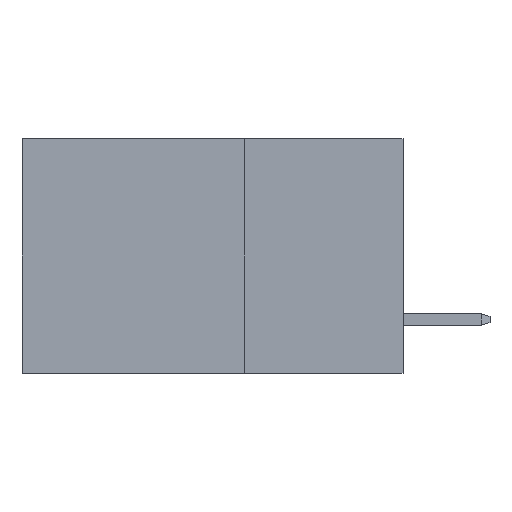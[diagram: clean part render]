
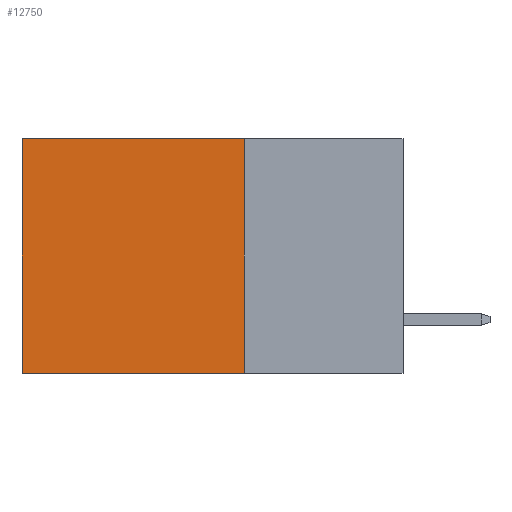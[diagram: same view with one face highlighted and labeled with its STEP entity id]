
A CAD part, left-side view. The second image highlights one B-rep face of the part: STEP entity #12750.
In plain terms, the highlighted planar face has unit normal (-1, 0, 0).
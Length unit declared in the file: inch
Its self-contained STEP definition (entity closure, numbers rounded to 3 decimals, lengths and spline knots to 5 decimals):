
#389 = VERTEX_POINT ( 'NONE', #21893 ) ;
#2027 = CARTESIAN_POINT ( 'NONE',  ( 0.2875, 0.25, 0. ) ) ;
#3282 = VECTOR ( 'NONE', #28069, 39.37008 ) ;
#3759 = EDGE_LOOP ( 'NONE', ( #11251, #27852, #19115, #13332 ) ) ;
#3894 = DIRECTION ( 'NONE',  ( 0., 0., -1. ) ) ;
#3931 = CARTESIAN_POINT ( 'NONE',  ( 0.2875, 0.25, 0. ) ) ;
#4018 = LINE ( 'NONE', #20995, #3282 ) ;
#4730 = EDGE_CURVE ( 'NONE', #18613, #8512, #9884, .T. ) ;
#5780 = DIRECTION ( 'NONE',  ( 0., 1., 0. ) ) ;
#8512 = VERTEX_POINT ( 'NONE', #23067 ) ;
#8759 = CARTESIAN_POINT ( 'NONE',  ( 0.2875, 0.6, 0. ) ) ;
#9617 = AXIS2_PLACEMENT_3D ( 'NONE', #3931, #10850, #17934 ) ;
#9884 = LINE ( 'NONE', #2027, #19022 ) ;
#10850 = DIRECTION ( 'NONE',  ( 1., 0., 0. ) ) ;
#11168 = CARTESIAN_POINT ( 'NONE',  ( 0.2875, 0.25, 0. ) ) ;
#11251 = ORIENTED_EDGE ( 'NONE', *, *, #18981, .T. ) ;
#12750 = ADVANCED_FACE ( 'NONE', ( #15571 ), #20440, .F. ) ;
#13332 = ORIENTED_EDGE ( 'NONE', *, *, #4730, .T. ) ;
#13730 = VECTOR ( 'NONE', #15968, 39.37008 ) ;
#14317 = VECTOR ( 'NONE', #3894, 39.37008 ) ;
#15013 = VERTEX_POINT ( 'NONE', #27443 ) ;
#15571 = FACE_OUTER_BOUND ( 'NONE', #3759, .T. ) ;
#15968 = DIRECTION ( 'NONE',  ( 0., 0., -1. ) ) ;
#16518 = EDGE_CURVE ( 'NONE', #18613, #389, #20830, .T. ) ;
#17934 = DIRECTION ( 'NONE',  ( 0., 0., -1. ) ) ;
#18613 = VERTEX_POINT ( 'NONE', #11168 ) ;
#18633 = CARTESIAN_POINT ( 'NONE',  ( 0.2875, 0.25, 0. ) ) ;
#18981 = EDGE_CURVE ( 'NONE', #8512, #15013, #25423, .T. ) ;
#19022 = VECTOR ( 'NONE', #5780, 39.37008 ) ;
#19055 = EDGE_CURVE ( 'NONE', #389, #15013, #4018, .T. ) ;
#19115 = ORIENTED_EDGE ( 'NONE', *, *, #16518, .F. ) ;
#20440 = PLANE ( 'NONE',  #9617 ) ;
#20830 = LINE ( 'NONE', #18633, #13730 ) ;
#20995 = CARTESIAN_POINT ( 'NONE',  ( 0.2875, 0.25, -0.37 ) ) ;
#21893 = CARTESIAN_POINT ( 'NONE',  ( 0.2875, 0.25, -0.37 ) ) ;
#23067 = CARTESIAN_POINT ( 'NONE',  ( 0.2875, 0.6, 0. ) ) ;
#25423 = LINE ( 'NONE', #8759, #14317 ) ;
#27443 = CARTESIAN_POINT ( 'NONE',  ( 0.2875, 0.6, -0.37 ) ) ;
#27852 = ORIENTED_EDGE ( 'NONE', *, *, #19055, .F. ) ;
#28069 = DIRECTION ( 'NONE',  ( 0., 1., 0. ) ) ;
